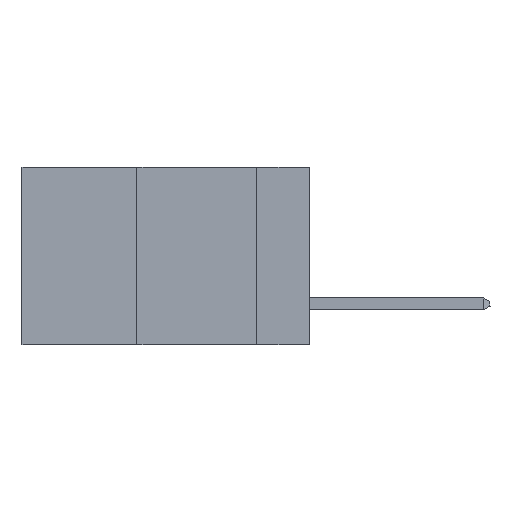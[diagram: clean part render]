
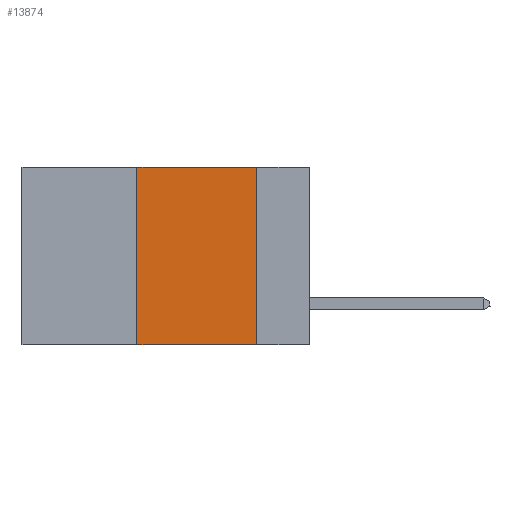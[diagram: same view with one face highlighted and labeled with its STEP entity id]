
A CAD part, left-side view. The second image highlights one B-rep face of the part: STEP entity #13874.
In plain terms, the highlighted planar face has unit normal (-1, 0, 0).
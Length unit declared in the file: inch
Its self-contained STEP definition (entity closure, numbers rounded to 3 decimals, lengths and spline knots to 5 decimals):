
#290 = DIRECTION ( 'NONE',  ( 1., 0., 0. ) ) ;
#318 = VECTOR ( 'NONE', #4075, 39.37008 ) ;
#603 = VERTEX_POINT ( 'NONE', #4037 ) ;
#991 = CARTESIAN_POINT ( 'NONE',  ( 0., 0.6, 0. ) ) ;
#1212 = EDGE_CURVE ( 'NONE', #603, #18349, #19117, .T. ) ;
#1354 = EDGE_CURVE ( 'NONE', #9482, #3303, #10607, .T. ) ;
#2169 = ORIENTED_EDGE ( 'NONE', *, *, #5803, .F. ) ;
#3303 = VERTEX_POINT ( 'NONE', #16846 ) ;
#3425 = VECTOR ( 'NONE', #19541, 39.37008 ) ;
#4037 = CARTESIAN_POINT ( 'NONE',  ( 0., 0.36, -0.37 ) ) ;
#4075 = DIRECTION ( 'NONE',  ( 0., -1., 0. ) ) ;
#4282 = CARTESIAN_POINT ( 'NONE',  ( 0., 0.11, 0. ) ) ;
#4727 = CARTESIAN_POINT ( 'NONE',  ( 0., 0.6, -0.37 ) ) ;
#5803 = EDGE_CURVE ( 'NONE', #18349, #9482, #8235, .T. ) ;
#6029 = VECTOR ( 'NONE', #8264, 39.37008 ) ;
#6093 = EDGE_CURVE ( 'NONE', #603, #3303, #15028, .T. ) ;
#7254 = EDGE_LOOP ( 'NONE', ( #18190, #2169, #17930, #7786 ) ) ;
#7786 = ORIENTED_EDGE ( 'NONE', *, *, #6093, .T. ) ;
#8235 = LINE ( 'NONE', #991, #318 ) ;
#8264 = DIRECTION ( 'NONE',  ( 0., -1., 0. ) ) ;
#9482 = VERTEX_POINT ( 'NONE', #12021 ) ;
#9492 = CARTESIAN_POINT ( 'NONE',  ( 0., 0.6, 0. ) ) ;
#10607 = LINE ( 'NONE', #4282, #12091 ) ;
#11314 = FACE_OUTER_BOUND ( 'NONE', #7254, .T. ) ;
#11366 = AXIS2_PLACEMENT_3D ( 'NONE', #9492, #290, #18818 ) ;
#12021 = CARTESIAN_POINT ( 'NONE',  ( 0., 0.11, 0. ) ) ;
#12091 = VECTOR ( 'NONE', #12694, 39.37008 ) ;
#12694 = DIRECTION ( 'NONE',  ( 0., 0., -1. ) ) ;
#13874 = ADVANCED_FACE ( 'NONE', ( #11314 ), #15662, .F. ) ;
#15028 = LINE ( 'NONE', #4727, #6029 ) ;
#15662 = PLANE ( 'NONE',  #11366 ) ;
#16846 = CARTESIAN_POINT ( 'NONE',  ( 0., 0.11, -0.37 ) ) ;
#17518 = CARTESIAN_POINT ( 'NONE',  ( 0., 0.36, 0. ) ) ;
#17930 = ORIENTED_EDGE ( 'NONE', *, *, #1212, .F. ) ;
#18120 = CARTESIAN_POINT ( 'NONE',  ( 0., 0.36, 0. ) ) ;
#18190 = ORIENTED_EDGE ( 'NONE', *, *, #1354, .F. ) ;
#18349 = VERTEX_POINT ( 'NONE', #17518 ) ;
#18818 = DIRECTION ( 'NONE',  ( 0., 0., -1. ) ) ;
#19117 = LINE ( 'NONE', #18120, #3425 ) ;
#19541 = DIRECTION ( 'NONE',  ( 0., 0., 1. ) ) ;
